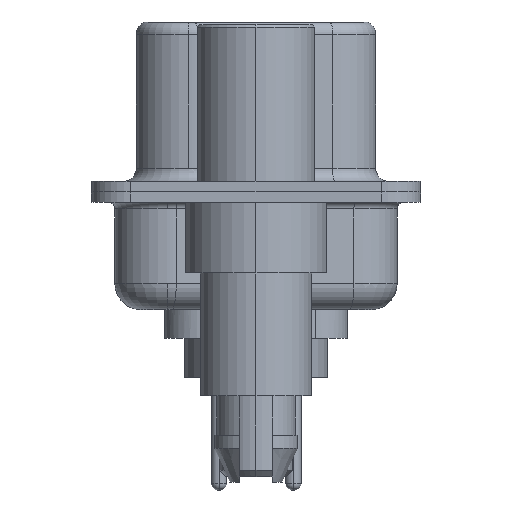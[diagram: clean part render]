
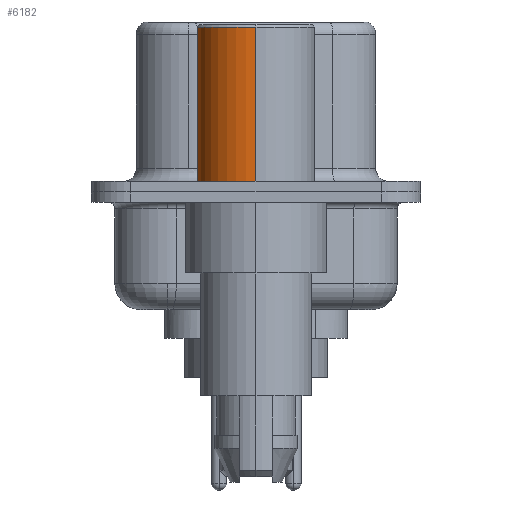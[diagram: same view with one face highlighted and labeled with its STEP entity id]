
A CAD part, left-side view. The second image highlights one B-rep face of the part: STEP entity #6182.
In plain terms, the highlighted cylindrical face has radius 2.25 mm (diameter 4.5 mm), a partial arc.
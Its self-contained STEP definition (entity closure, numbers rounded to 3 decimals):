
#992 = CARTESIAN_POINT ( 'NONE',  ( 2.25, 0., 6.3 ) ) ;
#1305 = EDGE_CURVE ( 'NONE', #13442, #17621, #6839, .T. ) ;
#1671 = DIRECTION ( 'NONE',  ( 1., 0., 0. ) ) ;
#1696 = LINE ( 'NONE', #8247, #13937 ) ;
#1812 = DIRECTION ( 'NONE',  ( 0., 0., 1. ) ) ;
#1849 = AXIS2_PLACEMENT_3D ( 'NONE', #16406, #2866, #20573 ) ;
#1880 = CARTESIAN_POINT ( 'NONE',  ( 0., 0., 6.3 ) ) ;
#1987 = EDGE_CURVE ( 'NONE', #13442, #13438, #8363, .T. ) ;
#2585 = CARTESIAN_POINT ( 'NONE',  ( 2.25, 0., 0.4 ) ) ;
#2866 = DIRECTION ( 'NONE',  ( 0., 0., 1. ) ) ;
#2932 = EDGE_CURVE ( 'NONE', #13438, #7533, #19290, .T. ) ;
#4476 = ORIENTED_EDGE ( 'NONE', *, *, #13090, .T. ) ;
#4835 = CARTESIAN_POINT ( 'NONE',  ( -2.25, 0., 0.4 ) ) ;
#5005 = DIRECTION ( 'NONE',  ( 0., 0., 1. ) ) ;
#5410 = CYLINDRICAL_SURFACE ( 'NONE', #1849, 2.25 ) ;
#6182 = ADVANCED_FACE ( 'NONE', ( #14366 ), #5410, .T. ) ;
#6839 = CIRCLE ( 'NONE', #16882, 2.25 ) ;
#7533 = VERTEX_POINT ( 'NONE', #8435 ) ;
#7810 = DIRECTION ( 'NONE',  ( 0., 0., 1. ) ) ;
#7859 = VECTOR ( 'NONE', #12869, 1000. ) ;
#8247 = CARTESIAN_POINT ( 'NONE',  ( -2.25, 0., 0.581 ) ) ;
#8363 = LINE ( 'NONE', #11590, #7859 ) ;
#8435 = CARTESIAN_POINT ( 'NONE',  ( -2.25, 0., 6.3 ) ) ;
#10294 = AXIS2_PLACEMENT_3D ( 'NONE', #1880, #1812, #1671 ) ;
#10961 = DIRECTION ( 'NONE',  ( 1., 0., 0. ) ) ;
#11590 = CARTESIAN_POINT ( 'NONE',  ( 2.25, 0., 0.581 ) ) ;
#11985 = ORIENTED_EDGE ( 'NONE', *, *, #1305, .T. ) ;
#12145 = CARTESIAN_POINT ( 'NONE',  ( 0., 0., 0.4 ) ) ;
#12869 = DIRECTION ( 'NONE',  ( 0., 0., 1. ) ) ;
#13090 = EDGE_CURVE ( 'NONE', #17621, #7533, #1696, .T. ) ;
#13438 = VERTEX_POINT ( 'NONE', #992 ) ;
#13442 = VERTEX_POINT ( 'NONE', #2585 ) ;
#13937 = VECTOR ( 'NONE', #5005, 1000. ) ;
#14366 = FACE_OUTER_BOUND ( 'NONE', #14709, .T. ) ;
#14662 = ORIENTED_EDGE ( 'NONE', *, *, #1987, .F. ) ;
#14709 = EDGE_LOOP ( 'NONE', ( #11985, #4476, #17518, #14662 ) ) ;
#16406 = CARTESIAN_POINT ( 'NONE',  ( 0., 0., 0.581 ) ) ;
#16882 = AXIS2_PLACEMENT_3D ( 'NONE', #12145, #7810, #10961 ) ;
#17518 = ORIENTED_EDGE ( 'NONE', *, *, #2932, .F. ) ;
#17621 = VERTEX_POINT ( 'NONE', #4835 ) ;
#19290 = CIRCLE ( 'NONE', #10294, 2.25 ) ;
#20573 = DIRECTION ( 'NONE',  ( 1., 0., 0. ) ) ;
